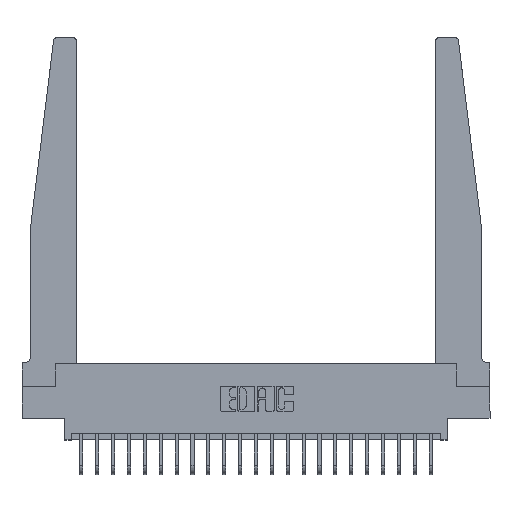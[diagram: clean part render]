
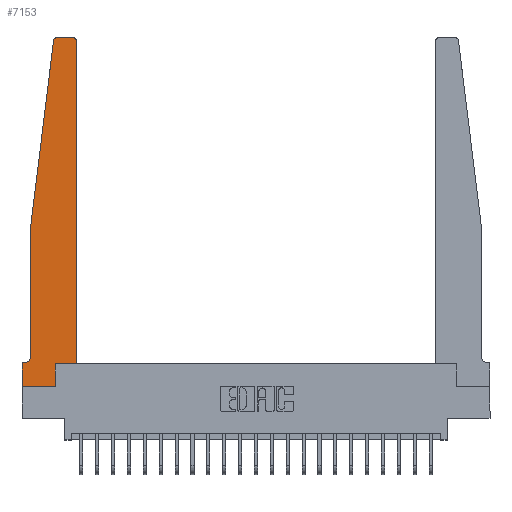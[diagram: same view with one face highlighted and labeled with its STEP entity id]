
A CAD part, top view. The second image highlights one B-rep face of the part: STEP entity #7153.
In plain terms, the highlighted planar face has unit normal (0, 0, 1).
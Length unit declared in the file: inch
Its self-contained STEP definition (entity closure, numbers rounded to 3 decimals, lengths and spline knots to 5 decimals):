
#469 = FACE_OUTER_BOUND ( 'NONE', #1139, .T. ) ;
#574 = VERTEX_POINT ( 'NONE', #1111 ) ;
#817 = DIRECTION ( 'NONE',  ( 1., 0., 0. ) ) ;
#827 = VERTEX_POINT ( 'NONE', #7158 ) ;
#1111 = CARTESIAN_POINT ( 'NONE',  ( 0.2605, 0.18, 0.37 ) ) ;
#1139 = EDGE_LOOP ( 'NONE', ( #8737, #8390, #3611, #15299, #10982, #4262, #4216, #15952, #16081, #3707, #1257, #18489 ) ) ;
#1165 = VERTEX_POINT ( 'NONE', #19802 ) ;
#1257 = ORIENTED_EDGE ( 'NONE', *, *, #18268, .T. ) ;
#1340 = DIRECTION ( 'NONE',  ( 0., 0., 1. ) ) ;
#1475 = AXIS2_PLACEMENT_3D ( 'NONE', #12068, #1955, #13767 ) ;
#1955 = DIRECTION ( 'NONE',  ( 0., 0., -1. ) ) ;
#2192 = CARTESIAN_POINT ( 'NONE',  ( 0., 0.1875, 0.37 ) ) ;
#2420 = EDGE_CURVE ( 'NONE', #4919, #574, #16875, .T. ) ;
#2691 = CARTESIAN_POINT ( 'NONE',  ( 0.065, 1.25, 0.37 ) ) ;
#2721 = CARTESIAN_POINT ( 'NONE',  ( 0.065, 1.25, 0.37 ) ) ;
#2838 = EDGE_CURVE ( 'NONE', #9099, #16209, #8405, .T. ) ;
#3611 = ORIENTED_EDGE ( 'NONE', *, *, #2838, .T. ) ;
#3707 = ORIENTED_EDGE ( 'NONE', *, *, #10334, .T. ) ;
#4102 = VERTEX_POINT ( 'NONE', #9522 ) ;
#4216 = ORIENTED_EDGE ( 'NONE', *, *, #18696, .T. ) ;
#4262 = ORIENTED_EDGE ( 'NONE', *, *, #8811, .T. ) ;
#4306 = CARTESIAN_POINT ( 'NONE',  ( 0.395, 2.72, 0.37 ) ) ;
#4332 = VECTOR ( 'NONE', #20398, 39.37008 ) ;
#4390 = DIRECTION ( 'NONE',  ( 0., -1., 0. ) ) ;
#4424 = DIRECTION ( 'NONE',  ( -0.122, -0.992, 0. ) ) ;
#4919 = VERTEX_POINT ( 'NONE', #8567 ) ;
#5378 = LINE ( 'NONE', #16356, #9315 ) ;
#5684 = LINE ( 'NONE', #7701, #14132 ) ;
#5857 = VECTOR ( 'NONE', #17898, 39.37008 ) ;
#5997 = DIRECTION ( 'NONE',  ( 1., 0., 0. ) ) ;
#6457 = CARTESIAN_POINT ( 'NONE',  ( 0.2605, 0.18, 0.37 ) ) ;
#6943 = CARTESIAN_POINT ( 'NONE',  ( 0.425, 0.18, 0.37 ) ) ;
#7153 = ADVANCED_FACE ( 'NONE', ( #469 ), #21514, .T. ) ;
#7158 = CARTESIAN_POINT ( 'NONE',  ( 0.27653, 2.75, 0.37 ) ) ;
#7701 = CARTESIAN_POINT ( 'NONE',  ( 0.065, 0.1875, 0.37 ) ) ;
#7747 = CARTESIAN_POINT ( 'NONE',  ( 0., 0., 0.37 ) ) ;
#7810 = VERTEX_POINT ( 'NONE', #15032 ) ;
#7867 = LINE ( 'NONE', #19151, #16303 ) ;
#7959 = DIRECTION ( 'NONE',  ( 0., -1., 0. ) ) ;
#8376 = VERTEX_POINT ( 'NONE', #9329 ) ;
#8390 = ORIENTED_EDGE ( 'NONE', *, *, #17844, .T. ) ;
#8405 = LINE ( 'NONE', #2721, #16854 ) ;
#8538 = CIRCLE ( 'NONE', #1475, 0.05 ) ;
#8567 = CARTESIAN_POINT ( 'NONE',  ( 0.2605, 0., 0.37 ) ) ;
#8680 = CARTESIAN_POINT ( 'NONE',  ( 0.425, 0.18, 0.37 ) ) ;
#8737 = ORIENTED_EDGE ( 'NONE', *, *, #15705, .T. ) ;
#8811 = EDGE_CURVE ( 'NONE', #8376, #15673, #5684, .T. ) ;
#8813 = LINE ( 'NONE', #2691, #21682 ) ;
#9056 = LINE ( 'NONE', #8680, #16441 ) ;
#9099 = VERTEX_POINT ( 'NONE', #16994 ) ;
#9315 = VECTOR ( 'NONE', #7959, 39.37008 ) ;
#9329 = CARTESIAN_POINT ( 'NONE',  ( 0.015, 0.1875, 0.37 ) ) ;
#9340 = LINE ( 'NONE', #6943, #4332 ) ;
#9414 = VERTEX_POINT ( 'NONE', #7747 ) ;
#9522 = CARTESIAN_POINT ( 'NONE',  ( 0.065, 0.2375, 0.37 ) ) ;
#10038 = EDGE_CURVE ( 'NONE', #16209, #4102, #8813, .T. ) ;
#10334 = EDGE_CURVE ( 'NONE', #574, #7810, #9056, .T. ) ;
#10336 = LINE ( 'NONE', #16199, #5857 ) ;
#10913 = DIRECTION ( 'NONE',  ( 0., 0., 1. ) ) ;
#10982 = ORIENTED_EDGE ( 'NONE', *, *, #18986, .T. ) ;
#11445 = DIRECTION ( 'NONE',  ( 0., 1., 0. ) ) ;
#12068 = CARTESIAN_POINT ( 'NONE',  ( 0.015, 0.2375, 0.37 ) ) ;
#13161 = DIRECTION ( 'NONE',  ( 1., 0., 0. ) ) ;
#13599 = CARTESIAN_POINT ( 'NONE',  ( 0.065, 1.25, 0.37 ) ) ;
#13767 = DIRECTION ( 'NONE',  ( -1., 0., 0. ) ) ;
#13771 = CARTESIAN_POINT ( 'NONE',  ( 0.425, 2.72, 0.37 ) ) ;
#14132 = VECTOR ( 'NONE', #16103, 39.37008 ) ;
#15032 = CARTESIAN_POINT ( 'NONE',  ( 0.425, 0.18, 0.37 ) ) ;
#15299 = ORIENTED_EDGE ( 'NONE', *, *, #10038, .T. ) ;
#15344 = AXIS2_PLACEMENT_3D ( 'NONE', #4306, #16096, #5997 ) ;
#15609 = VERTEX_POINT ( 'NONE', #13771 ) ;
#15673 = VERTEX_POINT ( 'NONE', #2192 ) ;
#15705 = EDGE_CURVE ( 'NONE', #1165, #827, #7867, .T. ) ;
#15952 = ORIENTED_EDGE ( 'NONE', *, *, #19502, .T. ) ;
#16081 = ORIENTED_EDGE ( 'NONE', *, *, #2420, .T. ) ;
#16096 = DIRECTION ( 'NONE',  ( 0., 0., 1. ) ) ;
#16103 = DIRECTION ( 'NONE',  ( -1., 0., 0. ) ) ;
#16199 = CARTESIAN_POINT ( 'NONE',  ( 0., 0., 0.37 ) ) ;
#16209 = VERTEX_POINT ( 'NONE', #13599 ) ;
#16303 = VECTOR ( 'NONE', #20807, 39.37008 ) ;
#16334 = VECTOR ( 'NONE', #11445, 39.37008 ) ;
#16356 = CARTESIAN_POINT ( 'NONE',  ( 0., 0., 0.37 ) ) ;
#16441 = VECTOR ( 'NONE', #17079, 39.37008 ) ;
#16854 = VECTOR ( 'NONE', #4424, 39.37008 ) ;
#16875 = LINE ( 'NONE', #6457, #16334 ) ;
#16994 = CARTESIAN_POINT ( 'NONE',  ( 0.24675, 2.72367, 0.37 ) ) ;
#17079 = DIRECTION ( 'NONE',  ( 1., 0., 0. ) ) ;
#17844 = EDGE_CURVE ( 'NONE', #827, #9099, #21727, .T. ) ;
#17898 = DIRECTION ( 'NONE',  ( 1., 0., 0. ) ) ;
#18173 = CARTESIAN_POINT ( 'NONE',  ( 0., 0.1875, 0.37 ) ) ;
#18268 = EDGE_CURVE ( 'NONE', #7810, #15609, #9340, .T. ) ;
#18489 = ORIENTED_EDGE ( 'NONE', *, *, #20071, .T. ) ;
#18696 = EDGE_CURVE ( 'NONE', #15673, #9414, #5378, .T. ) ;
#18986 = EDGE_CURVE ( 'NONE', #4102, #8376, #8538, .T. ) ;
#19011 = AXIS2_PLACEMENT_3D ( 'NONE', #20996, #10913, #817 ) ;
#19151 = CARTESIAN_POINT ( 'NONE',  ( 0.25, 2.75, 0.37 ) ) ;
#19502 = EDGE_CURVE ( 'NONE', #9414, #4919, #10336, .T. ) ;
#19802 = CARTESIAN_POINT ( 'NONE',  ( 0.395, 2.75, 0.37 ) ) ;
#20071 = EDGE_CURVE ( 'NONE', #15609, #1165, #21621, .T. ) ;
#20398 = DIRECTION ( 'NONE',  ( 0., 1., 0. ) ) ;
#20807 = DIRECTION ( 'NONE',  ( -1., 0., 0. ) ) ;
#20996 = CARTESIAN_POINT ( 'NONE',  ( 0.27653, 2.72, 0.37 ) ) ;
#21211 = AXIS2_PLACEMENT_3D ( 'NONE', #18173, #1340, #13161 ) ;
#21514 = PLANE ( 'NONE',  #21211 ) ;
#21621 = CIRCLE ( 'NONE', #15344, 0.03 ) ;
#21682 = VECTOR ( 'NONE', #4390, 39.37008 ) ;
#21727 = CIRCLE ( 'NONE', #19011, 0.03 ) ;
